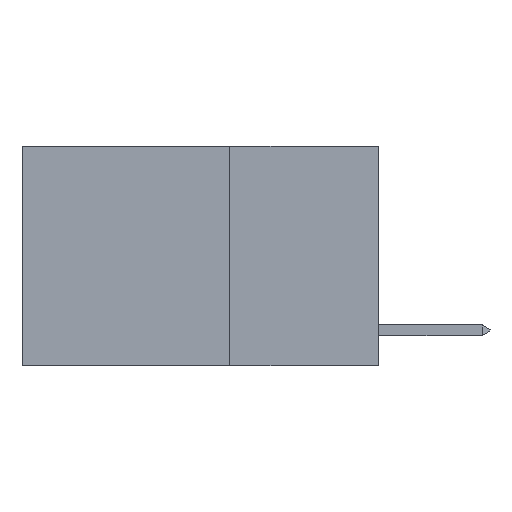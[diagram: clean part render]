
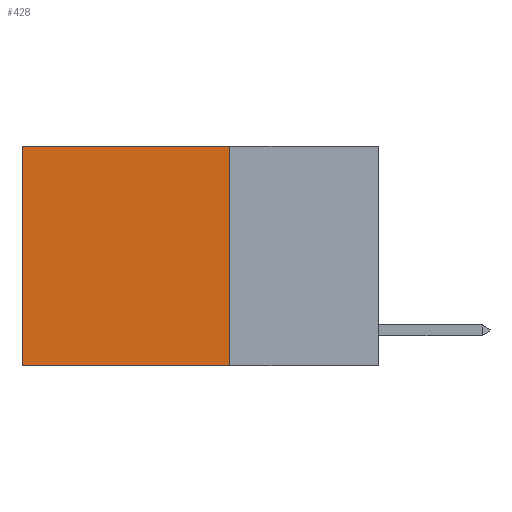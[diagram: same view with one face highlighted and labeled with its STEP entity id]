
A CAD part, left-side view. The second image highlights one B-rep face of the part: STEP entity #428.
In plain terms, the highlighted planar face has unit normal (-1, 0, 0).
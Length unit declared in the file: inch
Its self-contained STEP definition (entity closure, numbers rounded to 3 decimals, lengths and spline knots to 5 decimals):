
#117 = VERTEX_POINT ( 'NONE', #1914 ) ;
#262 = VECTOR ( 'NONE', #14372, 39.37008 ) ;
#428 = ADVANCED_FACE ( 'NONE', ( #10475 ), #8068, .F. ) ;
#881 = DIRECTION ( 'NONE',  ( 0., 1., 0. ) ) ;
#979 = ORIENTED_EDGE ( 'NONE', *, *, #10659, .F. ) ;
#984 = LINE ( 'NONE', #3180, #9742 ) ;
#1180 = VERTEX_POINT ( 'NONE', #1471 ) ;
#1471 = CARTESIAN_POINT ( 'NONE',  ( 0.2625, 0.6, -0.37 ) ) ;
#1474 = VECTOR ( 'NONE', #14533, 39.37008 ) ;
#1548 = EDGE_LOOP ( 'NONE', ( #10235, #979, #1673, #14702 ) ) ;
#1673 = ORIENTED_EDGE ( 'NONE', *, *, #10304, .F. ) ;
#1914 = CARTESIAN_POINT ( 'NONE',  ( 0.2625, 0.25, 0. ) ) ;
#2290 = LINE ( 'NONE', #12659, #8373 ) ;
#3180 = CARTESIAN_POINT ( 'NONE',  ( 0.2625, 0.25, 0. ) ) ;
#3340 = EDGE_CURVE ( 'NONE', #117, #8555, #984, .T. ) ;
#3370 = LINE ( 'NONE', #5346, #262 ) ;
#4868 = DIRECTION ( 'NONE',  ( 0., 0., -1. ) ) ;
#5346 = CARTESIAN_POINT ( 'NONE',  ( 0.2625, 0.25, -0.37 ) ) ;
#5502 = CARTESIAN_POINT ( 'NONE',  ( 0.2625, 0.6, 0. ) ) ;
#6382 = EDGE_CURVE ( 'NONE', #8555, #1180, #7201, .T. ) ;
#7201 = LINE ( 'NONE', #5502, #1474 ) ;
#7345 = CARTESIAN_POINT ( 'NONE',  ( 0.2625, 0.6, 0. ) ) ;
#7372 = AXIS2_PLACEMENT_3D ( 'NONE', #13432, #8922, #4868 ) ;
#7652 = VERTEX_POINT ( 'NONE', #10231 ) ;
#8068 = PLANE ( 'NONE',  #7372 ) ;
#8373 = VECTOR ( 'NONE', #9244, 39.37008 ) ;
#8555 = VERTEX_POINT ( 'NONE', #7345 ) ;
#8922 = DIRECTION ( 'NONE',  ( 1., 0., 0. ) ) ;
#9244 = DIRECTION ( 'NONE',  ( 0., 0., -1. ) ) ;
#9742 = VECTOR ( 'NONE', #881, 39.37008 ) ;
#10231 = CARTESIAN_POINT ( 'NONE',  ( 0.2625, 0.25, -0.37 ) ) ;
#10235 = ORIENTED_EDGE ( 'NONE', *, *, #6382, .T. ) ;
#10304 = EDGE_CURVE ( 'NONE', #117, #7652, #2290, .T. ) ;
#10475 = FACE_OUTER_BOUND ( 'NONE', #1548, .T. ) ;
#10659 = EDGE_CURVE ( 'NONE', #7652, #1180, #3370, .T. ) ;
#12659 = CARTESIAN_POINT ( 'NONE',  ( 0.2625, 0.25, 0. ) ) ;
#13432 = CARTESIAN_POINT ( 'NONE',  ( 0.2625, 0.25, 0. ) ) ;
#14372 = DIRECTION ( 'NONE',  ( 0., 1., 0. ) ) ;
#14533 = DIRECTION ( 'NONE',  ( 0., 0., -1. ) ) ;
#14702 = ORIENTED_EDGE ( 'NONE', *, *, #3340, .T. ) ;
